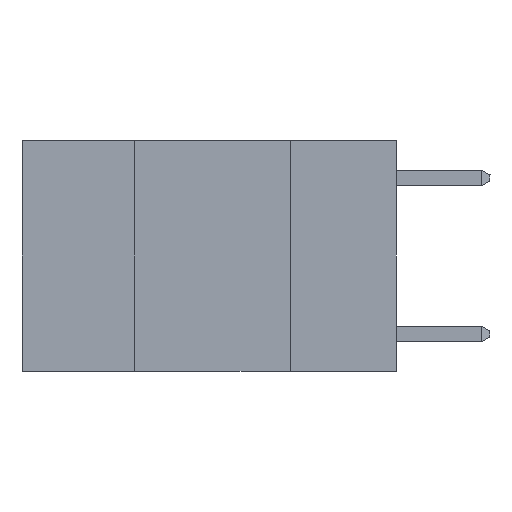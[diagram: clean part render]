
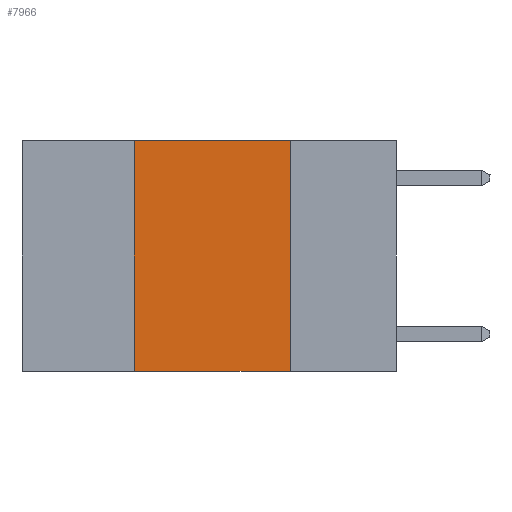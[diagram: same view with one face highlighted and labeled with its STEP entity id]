
A CAD part, left-side view. The second image highlights one B-rep face of the part: STEP entity #7966.
In plain terms, the highlighted planar face has unit normal (-1, 0, 0).
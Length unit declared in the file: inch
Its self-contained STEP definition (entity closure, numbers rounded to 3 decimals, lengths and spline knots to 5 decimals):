
#112 = CARTESIAN_POINT ( 'NONE',  ( 0., 0.17, -0.37 ) ) ;
#337 = DIRECTION ( 'NONE',  ( 0., 0., 1. ) ) ;
#1839 = ORIENTED_EDGE ( 'NONE', *, *, #8359, .F. ) ;
#2277 = ORIENTED_EDGE ( 'NONE', *, *, #13440, .F. ) ;
#2546 = CARTESIAN_POINT ( 'NONE',  ( 0., 0.42, 0. ) ) ;
#2681 = VERTEX_POINT ( 'NONE', #3123 ) ;
#3123 = CARTESIAN_POINT ( 'NONE',  ( 0., 0.17, 0. ) ) ;
#3133 = LINE ( 'NONE', #8273, #11349 ) ;
#3671 = DIRECTION ( 'NONE',  ( 0., 0., -1. ) ) ;
#3924 = VECTOR ( 'NONE', #3671, 39.37008 ) ;
#4011 = VERTEX_POINT ( 'NONE', #13363 ) ;
#4344 = PLANE ( 'NONE',  #9044 ) ;
#5435 = LINE ( 'NONE', #6077, #8414 ) ;
#5467 = DIRECTION ( 'NONE',  ( 1., 0., 0. ) ) ;
#5515 = DIRECTION ( 'NONE',  ( 0., -1., 0. ) ) ;
#5523 = ORIENTED_EDGE ( 'NONE', *, *, #5650, .F. ) ;
#5650 = EDGE_CURVE ( 'NONE', #4011, #10333, #3133, .T. ) ;
#5851 = EDGE_LOOP ( 'NONE', ( #2277, #1839, #5523, #10998 ) ) ;
#6077 = CARTESIAN_POINT ( 'NONE',  ( 0., 0.6, 0. ) ) ;
#7194 = DIRECTION ( 'NONE',  ( 0., -1., 0. ) ) ;
#7966 = ADVANCED_FACE ( 'NONE', ( #10348 ), #4344, .F. ) ;
#8273 = CARTESIAN_POINT ( 'NONE',  ( 0., 0.42, 0. ) ) ;
#8359 = EDGE_CURVE ( 'NONE', #10333, #2681, #5435, .T. ) ;
#8414 = VECTOR ( 'NONE', #7194, 39.37008 ) ;
#9044 = AXIS2_PLACEMENT_3D ( 'NONE', #12183, #5467, #13287 ) ;
#9431 = EDGE_CURVE ( 'NONE', #4011, #10969, #11525, .T. ) ;
#9872 = LINE ( 'NONE', #12632, #3924 ) ;
#10333 = VERTEX_POINT ( 'NONE', #2546 ) ;
#10348 = FACE_OUTER_BOUND ( 'NONE', #5851, .T. ) ;
#10969 = VERTEX_POINT ( 'NONE', #112 ) ;
#10998 = ORIENTED_EDGE ( 'NONE', *, *, #9431, .T. ) ;
#11349 = VECTOR ( 'NONE', #337, 39.37008 ) ;
#11525 = LINE ( 'NONE', #13399, #14507 ) ;
#12183 = CARTESIAN_POINT ( 'NONE',  ( 0., 0.6, 0. ) ) ;
#12632 = CARTESIAN_POINT ( 'NONE',  ( 0., 0.17, 0. ) ) ;
#13287 = DIRECTION ( 'NONE',  ( 0., 0., -1. ) ) ;
#13363 = CARTESIAN_POINT ( 'NONE',  ( 0., 0.42, -0.37 ) ) ;
#13399 = CARTESIAN_POINT ( 'NONE',  ( 0., 0.6, -0.37 ) ) ;
#13440 = EDGE_CURVE ( 'NONE', #2681, #10969, #9872, .T. ) ;
#14507 = VECTOR ( 'NONE', #5515, 39.37008 ) ;
